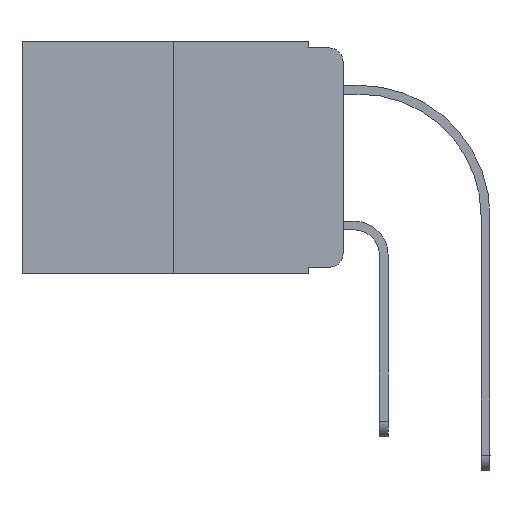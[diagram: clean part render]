
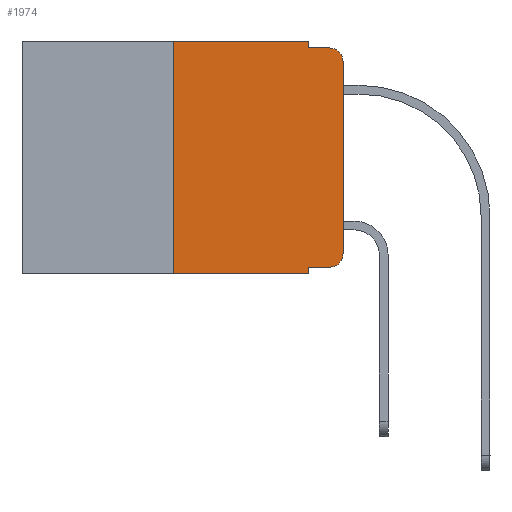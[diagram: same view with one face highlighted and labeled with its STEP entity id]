
A CAD part, left-side view. The second image highlights one B-rep face of the part: STEP entity #1974.
In plain terms, the highlighted planar face has unit normal (-1, 0, 0).
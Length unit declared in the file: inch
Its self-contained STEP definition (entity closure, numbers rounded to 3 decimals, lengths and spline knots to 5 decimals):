
#9 = ORIENTED_EDGE ( 'NONE', *, *, #8882, .F. ) ;
#425 = VERTEX_POINT ( 'NONE', #7109 ) ;
#622 = DIRECTION ( 'NONE',  ( 0., 0., -1. ) ) ;
#795 = CARTESIAN_POINT ( 'NONE',  ( 0., 0.02, -0.333 ) ) ;
#854 = VECTOR ( 'NONE', #12540, 39.37008 ) ;
#1178 = CARTESIAN_POINT ( 'NONE',  ( 0., 0.051, 0. ) ) ;
#1223 = ORIENTED_EDGE ( 'NONE', *, *, #11828, .F. ) ;
#1247 = CARTESIAN_POINT ( 'NONE',  ( 0., 0.25, 0. ) ) ;
#1860 = CARTESIAN_POINT ( 'NONE',  ( 0., 0.473, -0.343 ) ) ;
#1974 = ADVANCED_FACE ( 'NONE', ( #6515 ), #8618, .F. ) ;
#2262 = AXIS2_PLACEMENT_3D ( 'NONE', #11477, #2643, #622 ) ;
#2341 = AXIS2_PLACEMENT_3D ( 'NONE', #9901, #13101, #5218 ) ;
#2643 = DIRECTION ( 'NONE',  ( -1., 0., 0. ) ) ;
#2706 = VERTEX_POINT ( 'NONE', #13600 ) ;
#2802 = EDGE_CURVE ( 'NONE', #5748, #7924, #10891, .T. ) ;
#3903 = VERTEX_POINT ( 'NONE', #5285 ) ;
#4059 = LINE ( 'NONE', #7239, #6926 ) ;
#4106 = CARTESIAN_POINT ( 'NONE',  ( 0., 0.051, -0.333 ) ) ;
#4223 = VECTOR ( 'NONE', #7423, 39.37008 ) ;
#4413 = CARTESIAN_POINT ( 'NONE',  ( 0., 0.473, 0. ) ) ;
#4499 = ORIENTED_EDGE ( 'NONE', *, *, #6138, .T. ) ;
#4591 = CIRCLE ( 'NONE', #2262, 0.02 ) ;
#5070 = EDGE_CURVE ( 'NONE', #7894, #13384, #4591, .T. ) ;
#5168 = VERTEX_POINT ( 'NONE', #7204 ) ;
#5209 = DIRECTION ( 'NONE',  ( 0., -1., 0. ) ) ;
#5218 = DIRECTION ( 'NONE',  ( 0., 0., -1. ) ) ;
#5285 = CARTESIAN_POINT ( 'NONE',  ( 0., 0.25, 0. ) ) ;
#5311 = CARTESIAN_POINT ( 'NONE',  ( 0., 0.02, -0.01 ) ) ;
#5396 = DIRECTION ( 'NONE',  ( 0., 0., -1. ) ) ;
#5535 = ORIENTED_EDGE ( 'NONE', *, *, #8901, .F. ) ;
#5748 = VERTEX_POINT ( 'NONE', #6576 ) ;
#6120 = VERTEX_POINT ( 'NONE', #4106 ) ;
#6138 = EDGE_CURVE ( 'NONE', #425, #8313, #13411, .T. ) ;
#6235 = ORIENTED_EDGE ( 'NONE', *, *, #5070, .T. ) ;
#6284 = DIRECTION ( 'NONE',  ( 0., -1., 0. ) ) ;
#6515 = FACE_OUTER_BOUND ( 'NONE', #7039, .T. ) ;
#6576 = CARTESIAN_POINT ( 'NONE',  ( 0., 0.25, -0.343 ) ) ;
#6926 = VECTOR ( 'NONE', #5209, 39.37008 ) ;
#7039 = EDGE_LOOP ( 'NONE', ( #7378, #4499, #8647, #9, #1223, #5535, #12300, #7732, #8010, #6235 ) ) ;
#7089 = LINE ( 'NONE', #11291, #854 ) ;
#7109 = CARTESIAN_POINT ( 'NONE',  ( 0., 0., -0.03 ) ) ;
#7204 = CARTESIAN_POINT ( 'NONE',  ( 0., 0.051, -0.01 ) ) ;
#7208 = CARTESIAN_POINT ( 'NONE',  ( 0., 0.051, -0.01 ) ) ;
#7239 = CARTESIAN_POINT ( 'NONE',  ( 0., 0.051, -0.333 ) ) ;
#7378 = ORIENTED_EDGE ( 'NONE', *, *, #7572, .T. ) ;
#7423 = DIRECTION ( 'NONE',  ( 0., -1., 0. ) ) ;
#7572 = EDGE_CURVE ( 'NONE', #13384, #425, #12365, .T. ) ;
#7577 = VECTOR ( 'NONE', #6284, 39.37008 ) ;
#7732 = ORIENTED_EDGE ( 'NONE', *, *, #10755, .F. ) ;
#7829 = DIRECTION ( 'NONE',  ( 0., 0., 1. ) ) ;
#7894 = VERTEX_POINT ( 'NONE', #795 ) ;
#7924 = VERTEX_POINT ( 'NONE', #9616 ) ;
#8010 = ORIENTED_EDGE ( 'NONE', *, *, #12927, .T. ) ;
#8313 = VERTEX_POINT ( 'NONE', #5311 ) ;
#8523 = CARTESIAN_POINT ( 'NONE',  ( 0., 0.02, -0.03 ) ) ;
#8618 = PLANE ( 'NONE',  #2341 ) ;
#8647 = ORIENTED_EDGE ( 'NONE', *, *, #13839, .F. ) ;
#8696 = DIRECTION ( 'NONE',  ( 0., 0., -1. ) ) ;
#8774 = AXIS2_PLACEMENT_3D ( 'NONE', #8523, #11919, #5396 ) ;
#8863 = VECTOR ( 'NONE', #9109, 39.37008 ) ;
#8882 = EDGE_CURVE ( 'NONE', #2706, #5168, #8991, .T. ) ;
#8901 = EDGE_CURVE ( 'NONE', #5748, #3903, #10938, .T. ) ;
#8991 = LINE ( 'NONE', #1178, #12458 ) ;
#9109 = DIRECTION ( 'NONE',  ( 0., 0., 1. ) ) ;
#9471 = CARTESIAN_POINT ( 'NONE',  ( 0., 0., -0.313 ) ) ;
#9616 = CARTESIAN_POINT ( 'NONE',  ( 0., 0.051, -0.343 ) ) ;
#9901 = CARTESIAN_POINT ( 'NONE',  ( 0., 0.473, 0. ) ) ;
#10527 = DIRECTION ( 'NONE',  ( 0., -1., 0. ) ) ;
#10755 = EDGE_CURVE ( 'NONE', #6120, #7924, #7089, .T. ) ;
#10860 = VECTOR ( 'NONE', #10527, 39.37008 ) ;
#10891 = LINE ( 'NONE', #1860, #4223 ) ;
#10938 = LINE ( 'NONE', #1247, #13608 ) ;
#11265 = CARTESIAN_POINT ( 'NONE',  ( 0., 0., 0. ) ) ;
#11291 = CARTESIAN_POINT ( 'NONE',  ( 0., 0.051, 0. ) ) ;
#11477 = CARTESIAN_POINT ( 'NONE',  ( 0., 0.02, -0.313 ) ) ;
#11692 = LINE ( 'NONE', #7208, #10860 ) ;
#11828 = EDGE_CURVE ( 'NONE', #3903, #2706, #13088, .T. ) ;
#11919 = DIRECTION ( 'NONE',  ( -1., 0., 0. ) ) ;
#12300 = ORIENTED_EDGE ( 'NONE', *, *, #2802, .T. ) ;
#12365 = LINE ( 'NONE', #11265, #8863 ) ;
#12458 = VECTOR ( 'NONE', #8696, 39.37008 ) ;
#12540 = DIRECTION ( 'NONE',  ( 0., 0., -1. ) ) ;
#12927 = EDGE_CURVE ( 'NONE', #6120, #7894, #4059, .T. ) ;
#13088 = LINE ( 'NONE', #4413, #7577 ) ;
#13101 = DIRECTION ( 'NONE',  ( 1., 0., 0. ) ) ;
#13384 = VERTEX_POINT ( 'NONE', #9471 ) ;
#13411 = CIRCLE ( 'NONE', #8774, 0.02 ) ;
#13600 = CARTESIAN_POINT ( 'NONE',  ( 0., 0.051, 0. ) ) ;
#13608 = VECTOR ( 'NONE', #7829, 39.37008 ) ;
#13839 = EDGE_CURVE ( 'NONE', #5168, #8313, #11692, .T. ) ;
